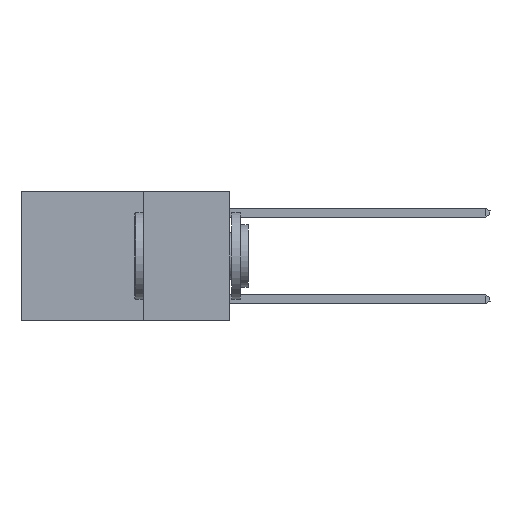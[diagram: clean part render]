
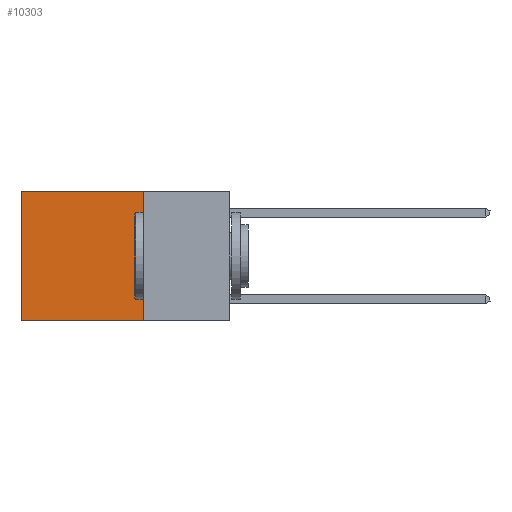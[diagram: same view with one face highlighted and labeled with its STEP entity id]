
A CAD part, left-side view. The second image highlights one B-rep face of the part: STEP entity #10303.
In plain terms, the highlighted planar face has unit normal (-1, 0, 0).
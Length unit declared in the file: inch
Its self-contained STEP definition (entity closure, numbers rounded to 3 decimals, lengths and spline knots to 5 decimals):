
#329 = DIRECTION ( 'NONE',  ( 0., 0., -1. ) ) ;
#644 = CARTESIAN_POINT ( 'NONE',  ( 0.2625, 0.25, -0.37 ) ) ;
#1012 = EDGE_CURVE ( 'NONE', #11865, #9034, #4537, .T. ) ;
#1232 = VECTOR ( 'NONE', #11559, 39.37008 ) ;
#2934 = CARTESIAN_POINT ( 'NONE',  ( 0.2625, 0.25, 0. ) ) ;
#3002 = EDGE_CURVE ( 'NONE', #11865, #13415, #4940, .T. ) ;
#3010 = LINE ( 'NONE', #644, #14637 ) ;
#4426 = VECTOR ( 'NONE', #7081, 39.37008 ) ;
#4537 = LINE ( 'NONE', #2934, #4426 ) ;
#4940 = LINE ( 'NONE', #13614, #5431 ) ;
#5077 = LINE ( 'NONE', #13994, #1232 ) ;
#5431 = VECTOR ( 'NONE', #16275, 39.37008 ) ;
#5813 = ORIENTED_EDGE ( 'NONE', *, *, #3002, .T. ) ;
#6179 = CARTESIAN_POINT ( 'NONE',  ( 0.2625, 0.25, 0. ) ) ;
#6940 = FACE_OUTER_BOUND ( 'NONE', #9975, .T. ) ;
#7081 = DIRECTION ( 'NONE',  ( 0., 0., -1. ) ) ;
#8342 = EDGE_CURVE ( 'NONE', #13415, #15943, #5077, .T. ) ;
#8612 = CARTESIAN_POINT ( 'NONE',  ( 0.2625, 0.25, -0.37 ) ) ;
#8677 = CARTESIAN_POINT ( 'NONE',  ( 0.2625, 0.6, -0.37 ) ) ;
#9034 = VERTEX_POINT ( 'NONE', #8612 ) ;
#9405 = CARTESIAN_POINT ( 'NONE',  ( 0.2625, 0.25, 0. ) ) ;
#9489 = DIRECTION ( 'NONE',  ( 1., 0., 0. ) ) ;
#9787 = ORIENTED_EDGE ( 'NONE', *, *, #1012, .F. ) ;
#9975 = EDGE_LOOP ( 'NONE', ( #13157, #13274, #9787, #5813 ) ) ;
#10303 = ADVANCED_FACE ( 'NONE', ( #6940 ), #13167, .F. ) ;
#10722 = DIRECTION ( 'NONE',  ( 0., 1., 0. ) ) ;
#11559 = DIRECTION ( 'NONE',  ( 0., 0., -1. ) ) ;
#11865 = VERTEX_POINT ( 'NONE', #6179 ) ;
#13157 = ORIENTED_EDGE ( 'NONE', *, *, #8342, .T. ) ;
#13167 = PLANE ( 'NONE',  #14042 ) ;
#13274 = ORIENTED_EDGE ( 'NONE', *, *, #14065, .F. ) ;
#13415 = VERTEX_POINT ( 'NONE', #13922 ) ;
#13614 = CARTESIAN_POINT ( 'NONE',  ( 0.2625, 0.25, 0. ) ) ;
#13922 = CARTESIAN_POINT ( 'NONE',  ( 0.2625, 0.6, 0. ) ) ;
#13994 = CARTESIAN_POINT ( 'NONE',  ( 0.2625, 0.6, 0. ) ) ;
#14042 = AXIS2_PLACEMENT_3D ( 'NONE', #9405, #9489, #329 ) ;
#14065 = EDGE_CURVE ( 'NONE', #9034, #15943, #3010, .T. ) ;
#14637 = VECTOR ( 'NONE', #10722, 39.37008 ) ;
#15943 = VERTEX_POINT ( 'NONE', #8677 ) ;
#16275 = DIRECTION ( 'NONE',  ( 0., 1., 0. ) ) ;
